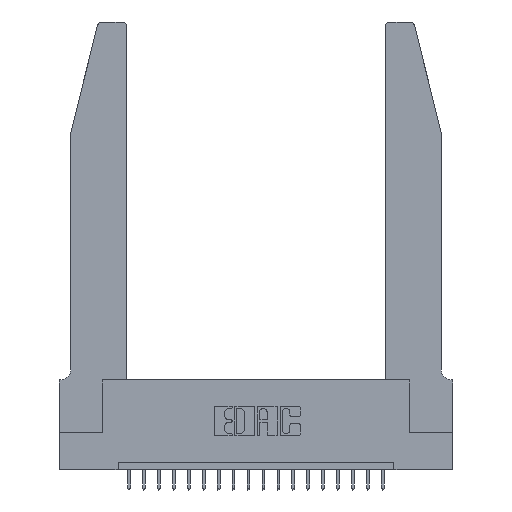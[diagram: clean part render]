
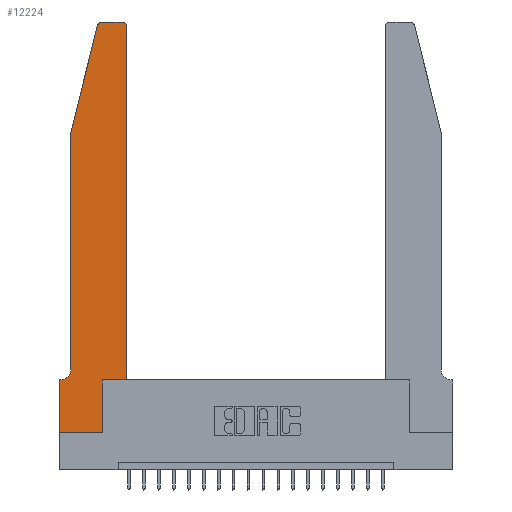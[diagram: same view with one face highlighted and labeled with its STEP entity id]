
A CAD part, top view. The second image highlights one B-rep face of the part: STEP entity #12224.
In plain terms, the highlighted planar face has unit normal (0, 0, 1).
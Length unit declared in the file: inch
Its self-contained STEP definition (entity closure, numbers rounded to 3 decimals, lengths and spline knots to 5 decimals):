
#36 = EDGE_LOOP ( 'NONE', ( #16092, #21041, #17305, #455, #2439, #12397, #4136, #2561, #20568, #19651, #6260, #10230 ) ) ;
#393 = CARTESIAN_POINT ( 'NONE',  ( 0.4505, 2.72, 0.37 ) ) ;
#455 = ORIENTED_EDGE ( 'NONE', *, *, #12245, .T. ) ;
#604 = CARTESIAN_POINT ( 'NONE',  ( 0., 0.35, 0.37 ) ) ;
#627 = CARTESIAN_POINT ( 'NONE',  ( 0.4505, 0.35, 0.37 ) ) ;
#903 = VECTOR ( 'NONE', #11572, 39.37008 ) ;
#997 = CARTESIAN_POINT ( 'NONE',  ( 0., 0., 0.37 ) ) ;
#1022 = LINE ( 'NONE', #11107, #11390 ) ;
#1415 = LINE ( 'NONE', #16103, #16031 ) ;
#2335 = EDGE_CURVE ( 'NONE', #2597, #10665, #6101, .T. ) ;
#2356 = VERTEX_POINT ( 'NONE', #10237 ) ;
#2439 = ORIENTED_EDGE ( 'NONE', *, *, #5516, .T. ) ;
#2561 = ORIENTED_EDGE ( 'NONE', *, *, #7711, .T. ) ;
#2597 = VERTEX_POINT ( 'NONE', #604 ) ;
#2664 = EDGE_CURVE ( 'NONE', #9400, #20808, #1022, .T. ) ;
#2848 = DIRECTION ( 'NONE',  ( 0., 0., 1. ) ) ;
#3374 = EDGE_CURVE ( 'NONE', #2356, #6786, #5889, .T. ) ;
#3609 = EDGE_CURVE ( 'NONE', #12987, #2597, #4899, .T. ) ;
#3678 = CARTESIAN_POINT ( 'NONE',  ( 0.0055, 0.35, 0.37 ) ) ;
#4136 = ORIENTED_EDGE ( 'NONE', *, *, #2335, .T. ) ;
#4179 = DIRECTION ( 'NONE',  ( -1., 0., 0. ) ) ;
#4274 = CARTESIAN_POINT ( 'NONE',  ( 0., 0.35, 0.37 ) ) ;
#4662 = DIRECTION ( 'NONE',  ( 0., 1., 0. ) ) ;
#4899 = LINE ( 'NONE', #13429, #903 ) ;
#5025 = VERTEX_POINT ( 'NONE', #16316 ) ;
#5516 = EDGE_CURVE ( 'NONE', #7099, #12987, #15280, .T. ) ;
#5889 = LINE ( 'NONE', #627, #12099 ) ;
#6101 = LINE ( 'NONE', #6203, #18028 ) ;
#6203 = CARTESIAN_POINT ( 'NONE',  ( 0., 0., 0.37 ) ) ;
#6230 = CARTESIAN_POINT ( 'NONE',  ( 0.0755, 2., 0.37 ) ) ;
#6260 = ORIENTED_EDGE ( 'NONE', *, *, #11963, .T. ) ;
#6299 = CARTESIAN_POINT ( 'NONE',  ( 0.4505, 0.35, 0.37 ) ) ;
#6470 = EDGE_CURVE ( 'NONE', #16722, #9400, #17755, .T. ) ;
#6672 = CIRCLE ( 'NONE', #8758, 0.03 ) ;
#6677 = VERTEX_POINT ( 'NONE', #19799 ) ;
#6724 = DIRECTION ( 'NONE',  ( 1., 0., 0. ) ) ;
#6786 = VERTEX_POINT ( 'NONE', #10996 ) ;
#7046 = CARTESIAN_POINT ( 'NONE',  ( 0.0055, 0.42, 0.37 ) ) ;
#7099 = VERTEX_POINT ( 'NONE', #13605 ) ;
#7177 = EDGE_CURVE ( 'NONE', #5025, #16722, #20815, .T. ) ;
#7307 = CARTESIAN_POINT ( 'NONE',  ( 0.284, 2.72, 0.37 ) ) ;
#7656 = FACE_OUTER_BOUND ( 'NONE', #36, .T. ) ;
#7711 = EDGE_CURVE ( 'NONE', #10665, #6677, #1415, .T. ) ;
#7869 = DIRECTION ( 'NONE',  ( 0., -1., 0. ) ) ;
#8455 = DIRECTION ( 'NONE',  ( 0., 0., 1. ) ) ;
#8758 = AXIS2_PLACEMENT_3D ( 'NONE', #13288, #8455, #6724 ) ;
#8932 = EDGE_CURVE ( 'NONE', #6677, #2356, #10807, .T. ) ;
#8936 = DIRECTION ( 'NONE',  ( 0., 1., 0. ) ) ;
#9063 = VECTOR ( 'NONE', #8936, 39.37008 ) ;
#9400 = VERTEX_POINT ( 'NONE', #18809 ) ;
#9706 = DIRECTION ( 'NONE',  ( 1., 0., 0. ) ) ;
#9971 = CARTESIAN_POINT ( 'NONE',  ( 0.284, 2.75, 0.37 ) ) ;
#10230 = ORIENTED_EDGE ( 'NONE', *, *, #10500, .T. ) ;
#10237 = CARTESIAN_POINT ( 'NONE',  ( 0.2865, 0.35, 0.37 ) ) ;
#10500 = EDGE_CURVE ( 'NONE', #21446, #5025, #6672, .T. ) ;
#10540 = CARTESIAN_POINT ( 'NONE',  ( 0.2605, 2.75, 0.37 ) ) ;
#10596 = CARTESIAN_POINT ( 'NONE',  ( 0.2865, 0.35, 0.37 ) ) ;
#10641 = DIRECTION ( 'NONE',  ( 0., 0., -1. ) ) ;
#10665 = VERTEX_POINT ( 'NONE', #997 ) ;
#10807 = LINE ( 'NONE', #10596, #9063 ) ;
#10996 = CARTESIAN_POINT ( 'NONE',  ( 0.4505, 0.35, 0.37 ) ) ;
#11107 = CARTESIAN_POINT ( 'NONE',  ( 0.0755, 2., 0.37 ) ) ;
#11390 = VECTOR ( 'NONE', #12171, 39.37008 ) ;
#11572 = DIRECTION ( 'NONE',  ( -1., 0., 0. ) ) ;
#11963 = EDGE_CURVE ( 'NONE', #6786, #21446, #16489, .T. ) ;
#12099 = VECTOR ( 'NONE', #12565, 39.37008 ) ;
#12171 = DIRECTION ( 'NONE',  ( -0.239, -0.971, 0. ) ) ;
#12224 = ADVANCED_FACE ( 'NONE', ( #7656 ), #21217, .T. ) ;
#12245 = EDGE_CURVE ( 'NONE', #20808, #7099, #14131, .T. ) ;
#12397 = ORIENTED_EDGE ( 'NONE', *, *, #3609, .T. ) ;
#12565 = DIRECTION ( 'NONE',  ( 1., 0., 0. ) ) ;
#12987 = VERTEX_POINT ( 'NONE', #3678 ) ;
#13288 = CARTESIAN_POINT ( 'NONE',  ( 0.4205, 2.72, 0.37 ) ) ;
#13322 = AXIS2_PLACEMENT_3D ( 'NONE', #4274, #2848, #19182 ) ;
#13429 = CARTESIAN_POINT ( 'NONE',  ( 0.0755, 0.35, 0.37 ) ) ;
#13605 = CARTESIAN_POINT ( 'NONE',  ( 0.0755, 0.42, 0.37 ) ) ;
#13654 = VECTOR ( 'NONE', #4662, 39.37008 ) ;
#14008 = DIRECTION ( 'NONE',  ( 0., 0., 1. ) ) ;
#14131 = LINE ( 'NONE', #21015, #21337 ) ;
#15280 = CIRCLE ( 'NONE', #20513, 0.07 ) ;
#15447 = DIRECTION ( 'NONE',  ( 1., 0., 0. ) ) ;
#15813 = DIRECTION ( 'NONE',  ( -1., 0., 0. ) ) ;
#16031 = VECTOR ( 'NONE', #9706, 39.37008 ) ;
#16071 = DIRECTION ( 'NONE',  ( 0., -1., 0. ) ) ;
#16092 = ORIENTED_EDGE ( 'NONE', *, *, #7177, .T. ) ;
#16103 = CARTESIAN_POINT ( 'NONE',  ( 0., 0., 0.37 ) ) ;
#16316 = CARTESIAN_POINT ( 'NONE',  ( 0.4205, 2.75, 0.37 ) ) ;
#16489 = LINE ( 'NONE', #6299, #13654 ) ;
#16722 = VERTEX_POINT ( 'NONE', #9971 ) ;
#16730 = VECTOR ( 'NONE', #4179, 39.37008 ) ;
#17305 = ORIENTED_EDGE ( 'NONE', *, *, #2664, .T. ) ;
#17755 = CIRCLE ( 'NONE', #19851, 0.03 ) ;
#18028 = VECTOR ( 'NONE', #16071, 39.37008 ) ;
#18809 = CARTESIAN_POINT ( 'NONE',  ( 0.25487, 2.72718, 0.37 ) ) ;
#19182 = DIRECTION ( 'NONE',  ( 1., 0., 0. ) ) ;
#19651 = ORIENTED_EDGE ( 'NONE', *, *, #3374, .T. ) ;
#19799 = CARTESIAN_POINT ( 'NONE',  ( 0.2865, 0., 0.37 ) ) ;
#19851 = AXIS2_PLACEMENT_3D ( 'NONE', #7307, #14008, #15447 ) ;
#20513 = AXIS2_PLACEMENT_3D ( 'NONE', #7046, #10641, #15813 ) ;
#20568 = ORIENTED_EDGE ( 'NONE', *, *, #8932, .T. ) ;
#20808 = VERTEX_POINT ( 'NONE', #6230 ) ;
#20815 = LINE ( 'NONE', #10540, #16730 ) ;
#21015 = CARTESIAN_POINT ( 'NONE',  ( 0.0755, 2., 0.37 ) ) ;
#21041 = ORIENTED_EDGE ( 'NONE', *, *, #6470, .T. ) ;
#21217 = PLANE ( 'NONE',  #13322 ) ;
#21337 = VECTOR ( 'NONE', #7869, 39.37008 ) ;
#21446 = VERTEX_POINT ( 'NONE', #393 ) ;
